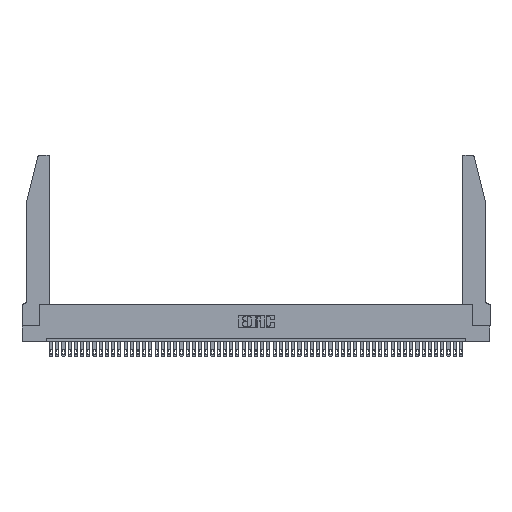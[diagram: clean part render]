
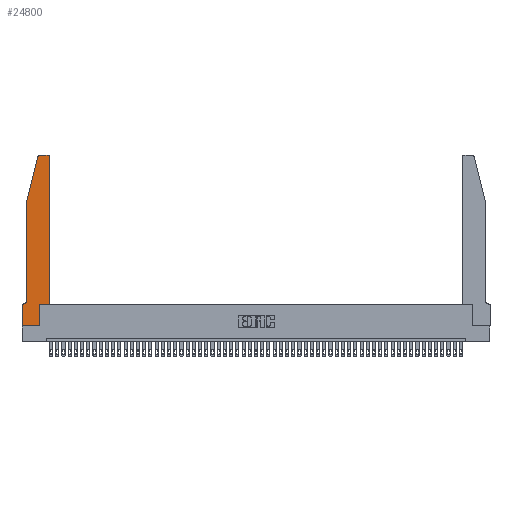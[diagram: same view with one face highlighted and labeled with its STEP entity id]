
A CAD part, top view. The second image highlights one B-rep face of the part: STEP entity #24800.
In plain terms, the highlighted planar face has unit normal (0, 0, 1).
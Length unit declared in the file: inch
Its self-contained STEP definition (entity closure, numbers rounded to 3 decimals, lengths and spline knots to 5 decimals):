
#303 = VECTOR ( 'NONE', #42115, 39.37008 ) ;
#481 = DIRECTION ( 'NONE',  ( 0., 1., 0. ) ) ;
#618 = LINE ( 'NONE', #46848, #9345 ) ;
#787 = CARTESIAN_POINT ( 'NONE',  ( 0.0755, 2., 0.37 ) ) ;
#1357 = LINE ( 'NONE', #787, #28231 ) ;
#1989 = PLANE ( 'NONE',  #32883 ) ;
#2724 = VERTEX_POINT ( 'NONE', #9092 ) ;
#2774 = DIRECTION ( 'NONE',  ( 1., 0., 0. ) ) ;
#3742 = LINE ( 'NONE', #16417, #39258 ) ;
#3960 = CARTESIAN_POINT ( 'NONE',  ( 0.4505, 2.72, 0.37 ) ) ;
#5431 = ORIENTED_EDGE ( 'NONE', *, *, #21133, .T. ) ;
#5833 = LINE ( 'NONE', #46641, #22003 ) ;
#6062 = CARTESIAN_POINT ( 'NONE',  ( 0.4505, 0.35, 0.37 ) ) ;
#6794 = DIRECTION ( 'NONE',  ( 0., 0., 1. ) ) ;
#7722 = EDGE_CURVE ( 'NONE', #50847, #40652, #24224, .T. ) ;
#8487 = ORIENTED_EDGE ( 'NONE', *, *, #13615, .T. ) ;
#9092 = CARTESIAN_POINT ( 'NONE',  ( 0.2865, 0., 0.37 ) ) ;
#9274 = CIRCLE ( 'NONE', #32215, 0.03 ) ;
#9345 = VECTOR ( 'NONE', #46653, 39.37008 ) ;
#9506 = VERTEX_POINT ( 'NONE', #35803 ) ;
#9547 = VERTEX_POINT ( 'NONE', #43288 ) ;
#12552 = DIRECTION ( 'NONE',  ( 0., 0., -1. ) ) ;
#13229 = ORIENTED_EDGE ( 'NONE', *, *, #21437, .T. ) ;
#13615 = EDGE_CURVE ( 'NONE', #40830, #43427, #39933, .T. ) ;
#13813 = LINE ( 'NONE', #50218, #18867 ) ;
#14127 = CARTESIAN_POINT ( 'NONE',  ( 0., 0., 0.37 ) ) ;
#14576 = DIRECTION ( 'NONE',  ( 0., 0., 1. ) ) ;
#14950 = CARTESIAN_POINT ( 'NONE',  ( 0.284, 2.72, 0.37 ) ) ;
#15476 = ORIENTED_EDGE ( 'NONE', *, *, #31958, .T. ) ;
#16417 = CARTESIAN_POINT ( 'NONE',  ( 0.0755, 0.35, 0.37 ) ) ;
#16450 = CARTESIAN_POINT ( 'NONE',  ( 0.0755, 0.42, 0.37 ) ) ;
#16646 = AXIS2_PLACEMENT_3D ( 'NONE', #39191, #12552, #40328 ) ;
#17062 = DIRECTION ( 'NONE',  ( -1., 0., 0. ) ) ;
#18637 = DIRECTION ( 'NONE',  ( 0., 1., 0. ) ) ;
#18867 = VECTOR ( 'NONE', #481, 39.37008 ) ;
#19215 = EDGE_CURVE ( 'NONE', #44890, #2724, #28418, .T. ) ;
#19976 = CARTESIAN_POINT ( 'NONE',  ( 0.284, 2.75, 0.37 ) ) ;
#20406 = VECTOR ( 'NONE', #17062, 39.37008 ) ;
#20632 = ORIENTED_EDGE ( 'NONE', *, *, #51052, .T. ) ;
#20710 = VERTEX_POINT ( 'NONE', #3960 ) ;
#21133 = EDGE_CURVE ( 'NONE', #42787, #20710, #5833, .T. ) ;
#21437 = EDGE_CURVE ( 'NONE', #47858, #9547, #1357, .T. ) ;
#21944 = EDGE_CURVE ( 'NONE', #43427, #9506, #3742, .T. ) ;
#22003 = VECTOR ( 'NONE', #18637, 39.37008 ) ;
#22710 = CARTESIAN_POINT ( 'NONE',  ( 0.0055, 0.35, 0.37 ) ) ;
#24224 = LINE ( 'NONE', #24595, #20406 ) ;
#24595 = CARTESIAN_POINT ( 'NONE',  ( 0.2605, 2.75, 0.37 ) ) ;
#24800 = ADVANCED_FACE ( 'NONE', ( #43721 ), #1989, .T. ) ;
#25427 = AXIS2_PLACEMENT_3D ( 'NONE', #14950, #14576, #42567 ) ;
#25708 = ORIENTED_EDGE ( 'NONE', *, *, #21944, .T. ) ;
#26139 = CARTESIAN_POINT ( 'NONE',  ( 0.4205, 2.72, 0.37 ) ) ;
#27861 = VECTOR ( 'NONE', #29972, 39.37008 ) ;
#28231 = VECTOR ( 'NONE', #51553, 39.37008 ) ;
#28418 = LINE ( 'NONE', #14127, #303 ) ;
#29362 = CIRCLE ( 'NONE', #25427, 0.03 ) ;
#29747 = CARTESIAN_POINT ( 'NONE',  ( 0., 0.35, 0.37 ) ) ;
#29804 = ORIENTED_EDGE ( 'NONE', *, *, #30350, .T. ) ;
#29972 = DIRECTION ( 'NONE',  ( 1., 0., 0. ) ) ;
#30119 = DIRECTION ( 'NONE',  ( 1., 0., 0. ) ) ;
#30295 = DIRECTION ( 'NONE',  ( 0., 0., 1. ) ) ;
#30350 = EDGE_CURVE ( 'NONE', #2724, #33057, #13813, .T. ) ;
#31958 = EDGE_CURVE ( 'NONE', #20710, #50847, #9274, .T. ) ;
#32215 = AXIS2_PLACEMENT_3D ( 'NONE', #26139, #6794, #2774 ) ;
#32816 = LINE ( 'NONE', #6062, #27861 ) ;
#32883 = AXIS2_PLACEMENT_3D ( 'NONE', #29747, #30295, #30119 ) ;
#33057 = VERTEX_POINT ( 'NONE', #42551 ) ;
#33373 = CARTESIAN_POINT ( 'NONE',  ( 0.4505, 0.35, 0.37 ) ) ;
#35403 = EDGE_CURVE ( 'NONE', #33057, #42787, #32816, .T. ) ;
#35803 = CARTESIAN_POINT ( 'NONE',  ( 0., 0.35, 0.37 ) ) ;
#36014 = DIRECTION ( 'NONE',  ( 0., -1., 0. ) ) ;
#36916 = DIRECTION ( 'NONE',  ( -1., 0., 0. ) ) ;
#37791 = ORIENTED_EDGE ( 'NONE', *, *, #50356, .T. ) ;
#38540 = EDGE_CURVE ( 'NONE', #9547, #40830, #45543, .T. ) ;
#39191 = CARTESIAN_POINT ( 'NONE',  ( 0.0055, 0.42, 0.37 ) ) ;
#39258 = VECTOR ( 'NONE', #36916, 39.37008 ) ;
#39523 = ORIENTED_EDGE ( 'NONE', *, *, #35403, .T. ) ;
#39933 = CIRCLE ( 'NONE', #16646, 0.07 ) ;
#40328 = DIRECTION ( 'NONE',  ( -1., 0., 0. ) ) ;
#40652 = VERTEX_POINT ( 'NONE', #19976 ) ;
#40830 = VERTEX_POINT ( 'NONE', #16450 ) ;
#41469 = CARTESIAN_POINT ( 'NONE',  ( 0.4205, 2.75, 0.37 ) ) ;
#42115 = DIRECTION ( 'NONE',  ( 1., 0., 0. ) ) ;
#42551 = CARTESIAN_POINT ( 'NONE',  ( 0.2865, 0.35, 0.37 ) ) ;
#42567 = DIRECTION ( 'NONE',  ( 1., 0., 0. ) ) ;
#42787 = VERTEX_POINT ( 'NONE', #33373 ) ;
#42905 = ORIENTED_EDGE ( 'NONE', *, *, #7722, .T. ) ;
#43288 = CARTESIAN_POINT ( 'NONE',  ( 0.0755, 2., 0.37 ) ) ;
#43427 = VERTEX_POINT ( 'NONE', #22710 ) ;
#43721 = FACE_OUTER_BOUND ( 'NONE', #47466, .T. ) ;
#44029 = CARTESIAN_POINT ( 'NONE',  ( 0.0755, 2., 0.37 ) ) ;
#44890 = VERTEX_POINT ( 'NONE', #48250 ) ;
#45543 = LINE ( 'NONE', #44029, #46869 ) ;
#46629 = ORIENTED_EDGE ( 'NONE', *, *, #38540, .T. ) ;
#46636 = ORIENTED_EDGE ( 'NONE', *, *, #19215, .T. ) ;
#46641 = CARTESIAN_POINT ( 'NONE',  ( 0.4505, 0.35, 0.37 ) ) ;
#46653 = DIRECTION ( 'NONE',  ( 0., -1., 0. ) ) ;
#46848 = CARTESIAN_POINT ( 'NONE',  ( 0., 0., 0.37 ) ) ;
#46869 = VECTOR ( 'NONE', #36014, 39.37008 ) ;
#47466 = EDGE_LOOP ( 'NONE', ( #42905, #20632, #13229, #46629, #8487, #25708, #37791, #46636, #29804, #39523, #5431, #15476 ) ) ;
#47738 = CARTESIAN_POINT ( 'NONE',  ( 0.25487, 2.72718, 0.37 ) ) ;
#47858 = VERTEX_POINT ( 'NONE', #47738 ) ;
#48250 = CARTESIAN_POINT ( 'NONE',  ( 0., 0., 0.37 ) ) ;
#50218 = CARTESIAN_POINT ( 'NONE',  ( 0.2865, 0.35, 0.37 ) ) ;
#50356 = EDGE_CURVE ( 'NONE', #9506, #44890, #618, .T. ) ;
#50847 = VERTEX_POINT ( 'NONE', #41469 ) ;
#51052 = EDGE_CURVE ( 'NONE', #40652, #47858, #29362, .T. ) ;
#51553 = DIRECTION ( 'NONE',  ( -0.239, -0.971, 0. ) ) ;
